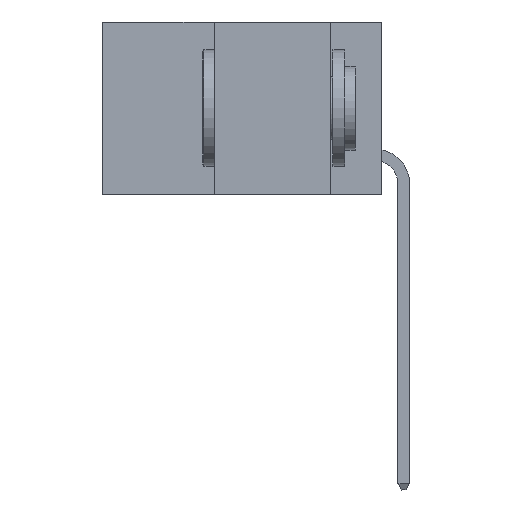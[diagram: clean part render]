
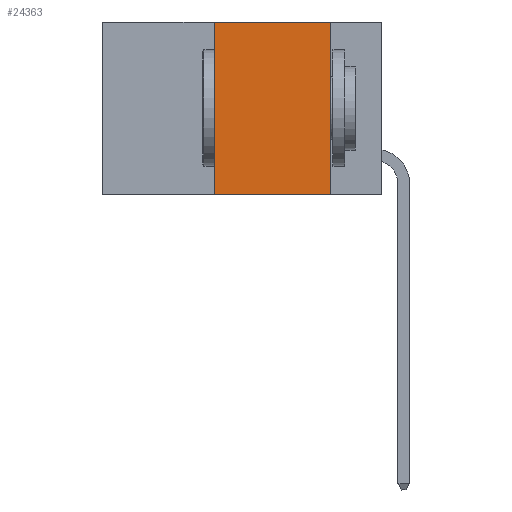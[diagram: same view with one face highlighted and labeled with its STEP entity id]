
A CAD part, left-side view. The second image highlights one B-rep face of the part: STEP entity #24363.
In plain terms, the highlighted planar face has unit normal (-1, 0, 0).
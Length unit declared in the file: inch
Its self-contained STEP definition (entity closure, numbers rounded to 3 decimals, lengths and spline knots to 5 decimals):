
#1570 = VECTOR ( 'NONE', #2225, 39.37008 ) ;
#2225 = DIRECTION ( 'NONE',  ( 0., -1., 0. ) ) ;
#2776 = VECTOR ( 'NONE', #4562, 39.37008 ) ;
#2990 = EDGE_CURVE ( 'NONE', #14259, #8378, #3874, .T. ) ;
#3225 = VECTOR ( 'NONE', #19564, 39.37008 ) ;
#3874 = LINE ( 'NONE', #21149, #3225 ) ;
#3894 = ORIENTED_EDGE ( 'NONE', *, *, #2990, .F. ) ;
#4562 = DIRECTION ( 'NONE',  ( 0., 0., 1. ) ) ;
#4894 = EDGE_CURVE ( 'NONE', #12573, #25748, #13793, .T. ) ;
#5285 = PLANE ( 'NONE',  #11270 ) ;
#6074 = CARTESIAN_POINT ( 'NONE',  ( 0., 0.11, 0. ) ) ;
#6493 = CARTESIAN_POINT ( 'NONE',  ( 0., 0.11, -0.37 ) ) ;
#6870 = DIRECTION ( 'NONE',  ( 0., -1., 0. ) ) ;
#7174 = LINE ( 'NONE', #20919, #1570 ) ;
#8238 = CARTESIAN_POINT ( 'NONE',  ( 0., 0.36, -0.37 ) ) ;
#8378 = VERTEX_POINT ( 'NONE', #6493 ) ;
#8640 = CARTESIAN_POINT ( 'NONE',  ( 0., 0.36, 0. ) ) ;
#8871 = CARTESIAN_POINT ( 'NONE',  ( 0., 0.6, 0. ) ) ;
#9366 = CARTESIAN_POINT ( 'NONE',  ( 0., 0.6, 0. ) ) ;
#9450 = DIRECTION ( 'NONE',  ( 1., 0., 0. ) ) ;
#11270 = AXIS2_PLACEMENT_3D ( 'NONE', #9366, #9450, #23902 ) ;
#11692 = ORIENTED_EDGE ( 'NONE', *, *, #23568, .F. ) ;
#12224 = CARTESIAN_POINT ( 'NONE',  ( 0., 0.36, 0. ) ) ;
#12573 = VERTEX_POINT ( 'NONE', #8238 ) ;
#13308 = ORIENTED_EDGE ( 'NONE', *, *, #13693, .T. ) ;
#13693 = EDGE_CURVE ( 'NONE', #12573, #8378, #7174, .T. ) ;
#13793 = LINE ( 'NONE', #8640, #2776 ) ;
#13826 = ORIENTED_EDGE ( 'NONE', *, *, #4894, .F. ) ;
#14259 = VERTEX_POINT ( 'NONE', #6074 ) ;
#15310 = VECTOR ( 'NONE', #6870, 39.37008 ) ;
#17025 = EDGE_LOOP ( 'NONE', ( #3894, #11692, #13826, #13308 ) ) ;
#19564 = DIRECTION ( 'NONE',  ( 0., 0., -1. ) ) ;
#20853 = LINE ( 'NONE', #8871, #15310 ) ;
#20919 = CARTESIAN_POINT ( 'NONE',  ( 0., 0.6, -0.37 ) ) ;
#21149 = CARTESIAN_POINT ( 'NONE',  ( 0., 0.11, 0. ) ) ;
#23568 = EDGE_CURVE ( 'NONE', #25748, #14259, #20853, .T. ) ;
#23902 = DIRECTION ( 'NONE',  ( 0., 0., -1. ) ) ;
#24028 = FACE_OUTER_BOUND ( 'NONE', #17025, .T. ) ;
#24363 = ADVANCED_FACE ( 'NONE', ( #24028 ), #5285, .F. ) ;
#25748 = VERTEX_POINT ( 'NONE', #12224 ) ;
